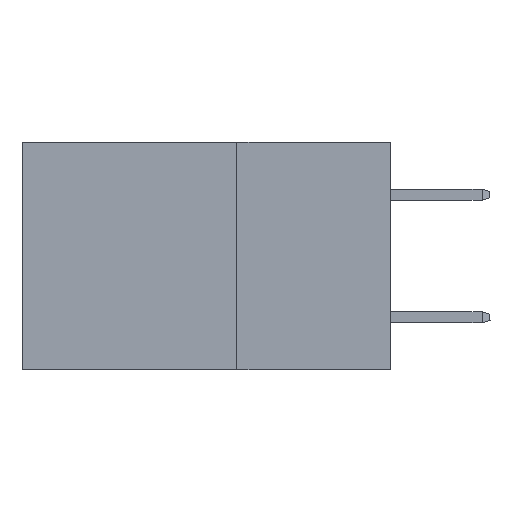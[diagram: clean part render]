
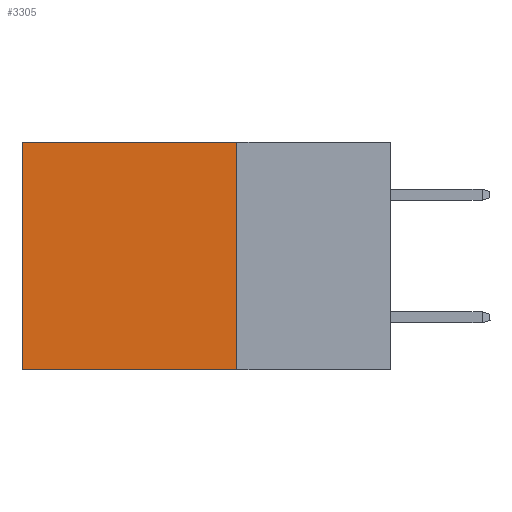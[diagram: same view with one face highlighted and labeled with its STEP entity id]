
A CAD part, left-side view. The second image highlights one B-rep face of the part: STEP entity #3305.
In plain terms, the highlighted planar face has unit normal (-1, 0, 0).
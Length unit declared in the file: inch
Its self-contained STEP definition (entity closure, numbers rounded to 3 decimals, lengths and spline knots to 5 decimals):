
#327 = CARTESIAN_POINT ( 'NONE',  ( 0.2875, 0.6, -0.37 ) ) ;
#849 = ORIENTED_EDGE ( 'NONE', *, *, #8807, .F. ) ;
#1213 = VECTOR ( 'NONE', #3336, 39.37008 ) ;
#1748 = VERTEX_POINT ( 'NONE', #19110 ) ;
#3305 = ADVANCED_FACE ( 'NONE', ( #25247 ), #28897, .F. ) ;
#3336 = DIRECTION ( 'NONE',  ( 0., 1., 0. ) ) ;
#3694 = AXIS2_PLACEMENT_3D ( 'NONE', #12614, #22108, #29094 ) ;
#3739 = LINE ( 'NONE', #27175, #17985 ) ;
#4350 = VERTEX_POINT ( 'NONE', #327 ) ;
#7878 = EDGE_CURVE ( 'NONE', #24108, #4350, #25369, .T. ) ;
#8807 = EDGE_CURVE ( 'NONE', #24313, #24108, #23489, .T. ) ;
#10506 = CARTESIAN_POINT ( 'NONE',  ( 0.2875, 0.25, -0.37 ) ) ;
#12614 = CARTESIAN_POINT ( 'NONE',  ( 0.2875, 0.25, 0. ) ) ;
#16078 = VECTOR ( 'NONE', #23123, 39.37008 ) ;
#17985 = VECTOR ( 'NONE', #24913, 39.37008 ) ;
#18000 = CARTESIAN_POINT ( 'NONE',  ( 0.2875, 0.25, -0.37 ) ) ;
#18806 = CARTESIAN_POINT ( 'NONE',  ( 0.2875, 0.25, 0. ) ) ;
#19110 = CARTESIAN_POINT ( 'NONE',  ( 0.2875, 0.6, 0. ) ) ;
#19213 = EDGE_CURVE ( 'NONE', #1748, #4350, #25581, .T. ) ;
#20112 = ORIENTED_EDGE ( 'NONE', *, *, #27858, .T. ) ;
#21798 = ORIENTED_EDGE ( 'NONE', *, *, #19213, .T. ) ;
#22108 = DIRECTION ( 'NONE',  ( 1., 0., 0. ) ) ;
#23123 = DIRECTION ( 'NONE',  ( 0., 0., -1. ) ) ;
#23489 = LINE ( 'NONE', #28148, #30069 ) ;
#23585 = EDGE_LOOP ( 'NONE', ( #21798, #28879, #849, #20112 ) ) ;
#24108 = VERTEX_POINT ( 'NONE', #18000 ) ;
#24313 = VERTEX_POINT ( 'NONE', #18806 ) ;
#24913 = DIRECTION ( 'NONE',  ( 0., 1., 0. ) ) ;
#25247 = FACE_OUTER_BOUND ( 'NONE', #23585, .T. ) ;
#25369 = LINE ( 'NONE', #10506, #1213 ) ;
#25581 = LINE ( 'NONE', #29780, #16078 ) ;
#25981 = DIRECTION ( 'NONE',  ( 0., 0., -1. ) ) ;
#27175 = CARTESIAN_POINT ( 'NONE',  ( 0.2875, 0.25, 0. ) ) ;
#27858 = EDGE_CURVE ( 'NONE', #24313, #1748, #3739, .T. ) ;
#28148 = CARTESIAN_POINT ( 'NONE',  ( 0.2875, 0.25, 0. ) ) ;
#28879 = ORIENTED_EDGE ( 'NONE', *, *, #7878, .F. ) ;
#28897 = PLANE ( 'NONE',  #3694 ) ;
#29094 = DIRECTION ( 'NONE',  ( 0., 0., -1. ) ) ;
#29780 = CARTESIAN_POINT ( 'NONE',  ( 0.2875, 0.6, 0. ) ) ;
#30069 = VECTOR ( 'NONE', #25981, 39.37008 ) ;
